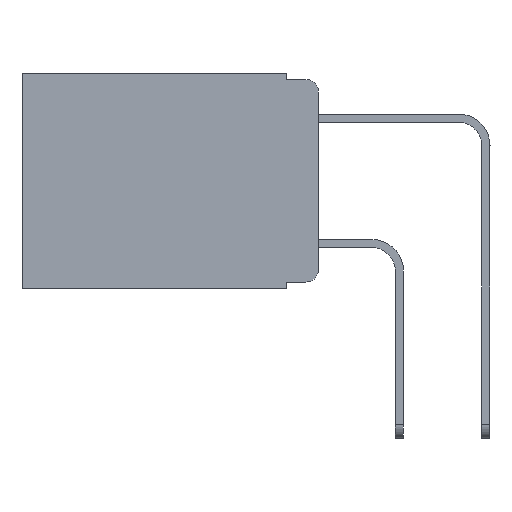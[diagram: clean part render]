
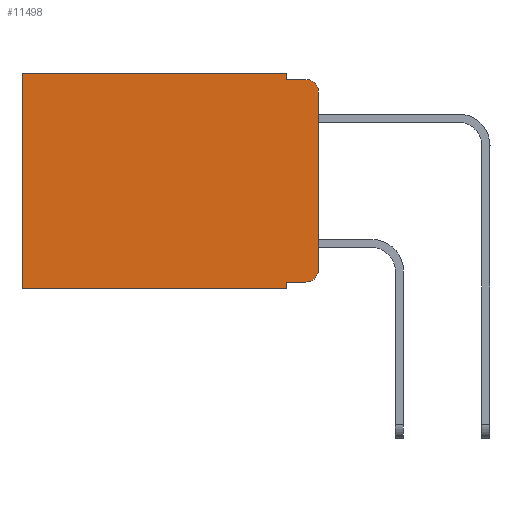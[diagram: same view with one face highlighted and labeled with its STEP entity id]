
A CAD part, left-side view. The second image highlights one B-rep face of the part: STEP entity #11498.
In plain terms, the highlighted planar face has unit normal (-1, 0, 0).
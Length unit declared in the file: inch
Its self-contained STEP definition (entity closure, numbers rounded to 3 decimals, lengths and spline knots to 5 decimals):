
#824 = CARTESIAN_POINT ( 'NONE',  ( 0.298, 0., -0.313 ) ) ;
#908 = LINE ( 'NONE', #3128, #10108 ) ;
#915 = ORIENTED_EDGE ( 'NONE', *, *, #6533, .F. ) ;
#962 = EDGE_CURVE ( 'NONE', #7054, #4865, #10288, .T. ) ;
#1380 = LINE ( 'NONE', #9186, #10016 ) ;
#1605 = VERTEX_POINT ( 'NONE', #5606 ) ;
#1646 = ORIENTED_EDGE ( 'NONE', *, *, #9233, .T. ) ;
#1673 = LINE ( 'NONE', #10805, #4810 ) ;
#1755 = DIRECTION ( 'NONE',  ( 0., 1., 0. ) ) ;
#2007 = DIRECTION ( 'NONE',  ( 0., 0., -1. ) ) ;
#2029 = DIRECTION ( 'NONE',  ( 0., 0., -1. ) ) ;
#2084 = CARTESIAN_POINT ( 'NONE',  ( 0.298, 0.051, -0.343 ) ) ;
#2114 = EDGE_CURVE ( 'NONE', #5459, #1605, #5747, .T. ) ;
#2332 = ORIENTED_EDGE ( 'NONE', *, *, #7735, .F. ) ;
#2514 = PLANE ( 'NONE',  #8020 ) ;
#2573 = VERTEX_POINT ( 'NONE', #6360 ) ;
#2907 = DIRECTION ( 'NONE',  ( -1., 0., 0. ) ) ;
#3026 = ORIENTED_EDGE ( 'NONE', *, *, #5447, .F. ) ;
#3128 = CARTESIAN_POINT ( 'NONE',  ( 0.298, 0.051, -0.01 ) ) ;
#3236 = ORIENTED_EDGE ( 'NONE', *, *, #2114, .T. ) ;
#3264 = EDGE_CURVE ( 'NONE', #4865, #2573, #5331, .T. ) ;
#3291 = CARTESIAN_POINT ( 'NONE',  ( 0.298, 0.02, -0.01 ) ) ;
#3615 = DIRECTION ( 'NONE',  ( 0., 1., 0. ) ) ;
#3681 = CARTESIAN_POINT ( 'NONE',  ( 0.298, 0.02, -0.313 ) ) ;
#3949 = LINE ( 'NONE', #11062, #10010 ) ;
#4161 = CARTESIAN_POINT ( 'NONE',  ( 0.298, 0.051, 0. ) ) ;
#4328 = CARTESIAN_POINT ( 'NONE',  ( 0.298, 0.473, 0. ) ) ;
#4365 = DIRECTION ( 'NONE',  ( 0., 0., -1. ) ) ;
#4423 = CARTESIAN_POINT ( 'NONE',  ( 0.298, 0., 0. ) ) ;
#4810 = VECTOR ( 'NONE', #1755, 39.37008 ) ;
#4851 = CIRCLE ( 'NONE', #9351, 0.02 ) ;
#4865 = VERTEX_POINT ( 'NONE', #8035 ) ;
#5084 = VECTOR ( 'NONE', #3615, 39.37008 ) ;
#5154 = EDGE_CURVE ( 'NONE', #10358, #8415, #908, .T. ) ;
#5331 = LINE ( 'NONE', #4328, #10715 ) ;
#5399 = LINE ( 'NONE', #4161, #6840 ) ;
#5447 = EDGE_CURVE ( 'NONE', #5459, #7382, #3949, .T. ) ;
#5459 = VERTEX_POINT ( 'NONE', #7384 ) ;
#5606 = CARTESIAN_POINT ( 'NONE',  ( 0.298, 0.02, -0.333 ) ) ;
#5747 = LINE ( 'NONE', #10576, #7308 ) ;
#6000 = DIRECTION ( 'NONE',  ( 0., -1., 0. ) ) ;
#6098 = EDGE_CURVE ( 'NONE', #1605, #11478, #4851, .T. ) ;
#6360 = CARTESIAN_POINT ( 'NONE',  ( 0.298, 0.473, -0.343 ) ) ;
#6533 = EDGE_CURVE ( 'NONE', #7054, #10358, #5399, .T. ) ;
#6840 = VECTOR ( 'NONE', #7824, 39.37008 ) ;
#7054 = VERTEX_POINT ( 'NONE', #7296 ) ;
#7092 = ORIENTED_EDGE ( 'NONE', *, *, #962, .T. ) ;
#7142 = DIRECTION ( 'NONE',  ( 0., -1., 0. ) ) ;
#7296 = CARTESIAN_POINT ( 'NONE',  ( 0.298, 0.051, 0. ) ) ;
#7308 = VECTOR ( 'NONE', #7142, 39.37008 ) ;
#7311 = DIRECTION ( 'NONE',  ( 0., 0., -1. ) ) ;
#7322 = CARTESIAN_POINT ( 'NONE',  ( 0.298, 0., -0.03 ) ) ;
#7369 = ORIENTED_EDGE ( 'NONE', *, *, #3264, .T. ) ;
#7382 = VERTEX_POINT ( 'NONE', #2084 ) ;
#7384 = CARTESIAN_POINT ( 'NONE',  ( 0.298, 0.051, -0.333 ) ) ;
#7552 = ORIENTED_EDGE ( 'NONE', *, *, #6098, .T. ) ;
#7735 = EDGE_CURVE ( 'NONE', #7382, #2573, #1673, .T. ) ;
#7824 = DIRECTION ( 'NONE',  ( 0., 0., -1. ) ) ;
#7860 = AXIS2_PLACEMENT_3D ( 'NONE', #8119, #9809, #7961 ) ;
#7952 = ORIENTED_EDGE ( 'NONE', *, *, #8151, .F. ) ;
#7961 = DIRECTION ( 'NONE',  ( 0., 0., -1. ) ) ;
#8020 = AXIS2_PLACEMENT_3D ( 'NONE', #4423, #10718, #8847 ) ;
#8035 = CARTESIAN_POINT ( 'NONE',  ( 0.298, 0.473, 0. ) ) ;
#8119 = CARTESIAN_POINT ( 'NONE',  ( 0.298, 0.02, -0.03 ) ) ;
#8151 = EDGE_CURVE ( 'NONE', #9942, #11478, #1380, .T. ) ;
#8415 = VERTEX_POINT ( 'NONE', #3291 ) ;
#8847 = DIRECTION ( 'NONE',  ( 0., 0., -1. ) ) ;
#9186 = CARTESIAN_POINT ( 'NONE',  ( 0.298, 0., 0. ) ) ;
#9233 = EDGE_CURVE ( 'NONE', #9942, #8415, #10192, .T. ) ;
#9351 = AXIS2_PLACEMENT_3D ( 'NONE', #3681, #2907, #7311 ) ;
#9755 = CARTESIAN_POINT ( 'NONE',  ( 0.298, 0.051, -0.01 ) ) ;
#9809 = DIRECTION ( 'NONE',  ( -1., 0., 0. ) ) ;
#9840 = CARTESIAN_POINT ( 'NONE',  ( 0.298, 0., 0. ) ) ;
#9942 = VERTEX_POINT ( 'NONE', #7322 ) ;
#10010 = VECTOR ( 'NONE', #2029, 39.37008 ) ;
#10016 = VECTOR ( 'NONE', #2007, 39.37008 ) ;
#10108 = VECTOR ( 'NONE', #6000, 39.37008 ) ;
#10148 = FACE_OUTER_BOUND ( 'NONE', #11200, .T. ) ;
#10192 = CIRCLE ( 'NONE', #7860, 0.02 ) ;
#10288 = LINE ( 'NONE', #9840, #5084 ) ;
#10358 = VERTEX_POINT ( 'NONE', #9755 ) ;
#10576 = CARTESIAN_POINT ( 'NONE',  ( 0.298, 0.051, -0.333 ) ) ;
#10715 = VECTOR ( 'NONE', #4365, 39.37008 ) ;
#10718 = DIRECTION ( 'NONE',  ( 1., 0., 0. ) ) ;
#10805 = CARTESIAN_POINT ( 'NONE',  ( 0.298, 0., -0.343 ) ) ;
#11062 = CARTESIAN_POINT ( 'NONE',  ( 0.298, 0.051, 0. ) ) ;
#11200 = EDGE_LOOP ( 'NONE', ( #7952, #1646, #11270, #915, #7092, #7369, #2332, #3026, #3236, #7552 ) ) ;
#11270 = ORIENTED_EDGE ( 'NONE', *, *, #5154, .F. ) ;
#11478 = VERTEX_POINT ( 'NONE', #824 ) ;
#11498 = ADVANCED_FACE ( 'NONE', ( #10148 ), #2514, .F. ) ;
